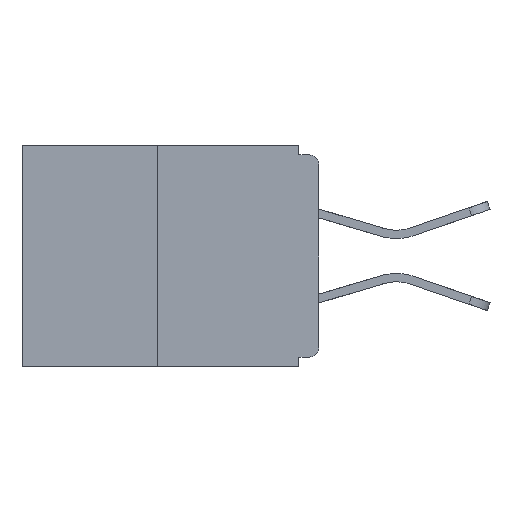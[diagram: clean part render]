
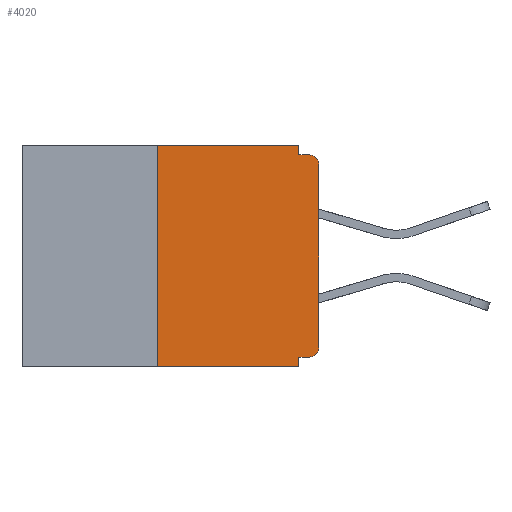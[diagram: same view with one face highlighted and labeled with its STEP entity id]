
A CAD part, left-side view. The second image highlights one B-rep face of the part: STEP entity #4020.
In plain terms, the highlighted planar face has unit normal (-1, 0, 0).
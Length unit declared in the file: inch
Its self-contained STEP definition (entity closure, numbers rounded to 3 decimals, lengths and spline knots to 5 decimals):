
#29 = VERTEX_POINT ( 'NONE', #1509 ) ;
#226 = DIRECTION ( 'NONE',  ( -1., 0., 0. ) ) ;
#231 = CARTESIAN_POINT ( 'NONE',  ( 0., 0.46, -0.343 ) ) ;
#475 = ORIENTED_EDGE ( 'NONE', *, *, #24253, .T. ) ;
#1274 = CARTESIAN_POINT ( 'NONE',  ( 0., 0., -0.015 ) ) ;
#1509 = CARTESIAN_POINT ( 'NONE',  ( 0., 0.015, -0.328 ) ) ;
#2218 = EDGE_CURVE ( 'NONE', #24492, #15950, #18961, .T. ) ;
#2872 = ORIENTED_EDGE ( 'NONE', *, *, #11935, .F. ) ;
#3116 = CARTESIAN_POINT ( 'NONE',  ( 0., 0.25, 0. ) ) ;
#3188 = CARTESIAN_POINT ( 'NONE',  ( 0., 0.25, 0. ) ) ;
#3460 = CARTESIAN_POINT ( 'NONE',  ( 0., 0.46, 0. ) ) ;
#3694 = DIRECTION ( 'NONE',  ( 0., 0., -1. ) ) ;
#4020 = ADVANCED_FACE ( 'NONE', ( #11728 ), #17610, .F. ) ;
#4146 = ORIENTED_EDGE ( 'NONE', *, *, #2218, .T. ) ;
#4351 = LINE ( 'NONE', #231, #6164 ) ;
#4354 = VERTEX_POINT ( 'NONE', #24860 ) ;
#5093 = CARTESIAN_POINT ( 'NONE',  ( 0., 0., -0.03 ) ) ;
#5268 = VECTOR ( 'NONE', #15161, 39.37008 ) ;
#5299 = LINE ( 'NONE', #11426, #5268 ) ;
#6164 = VECTOR ( 'NONE', #14494, 39.37008 ) ;
#6224 = CARTESIAN_POINT ( 'NONE',  ( 0., 0.25, -0.343 ) ) ;
#6852 = CARTESIAN_POINT ( 'NONE',  ( 0., 0., -0.328 ) ) ;
#7406 = LINE ( 'NONE', #1274, #23758 ) ;
#8199 = AXIS2_PLACEMENT_3D ( 'NONE', #9554, #17710, #3694 ) ;
#9290 = EDGE_CURVE ( 'NONE', #18717, #4354, #5299, .T. ) ;
#9554 = CARTESIAN_POINT ( 'NONE',  ( 0., 0.015, -0.313 ) ) ;
#9602 = VECTOR ( 'NONE', #14919, 39.37008 ) ;
#9695 = VERTEX_POINT ( 'NONE', #20982 ) ;
#9740 = DIRECTION ( 'NONE',  ( 0., 0., -1. ) ) ;
#9750 = CARTESIAN_POINT ( 'NONE',  ( 0., 0.031, 0. ) ) ;
#10863 = AXIS2_PLACEMENT_3D ( 'NONE', #3460, #19730, #9740 ) ;
#11277 = VERTEX_POINT ( 'NONE', #6224 ) ;
#11426 = CARTESIAN_POINT ( 'NONE',  ( 0., 0.031, 0. ) ) ;
#11728 = FACE_OUTER_BOUND ( 'NONE', #16400, .T. ) ;
#11935 = EDGE_CURVE ( 'NONE', #14613, #18717, #23924, .T. ) ;
#12484 = EDGE_CURVE ( 'NONE', #4354, #17338, #7406, .T. ) ;
#12827 = DIRECTION ( 'NONE',  ( 0., 0., 1. ) ) ;
#13901 = ORIENTED_EDGE ( 'NONE', *, *, #18565, .F. ) ;
#14037 = ORIENTED_EDGE ( 'NONE', *, *, #12484, .F. ) ;
#14494 = DIRECTION ( 'NONE',  ( 0., -1., 0. ) ) ;
#14555 = ORIENTED_EDGE ( 'NONE', *, *, #15553, .F. ) ;
#14613 = VERTEX_POINT ( 'NONE', #3188 ) ;
#14919 = DIRECTION ( 'NONE',  ( 0., 0., -1. ) ) ;
#15161 = DIRECTION ( 'NONE',  ( 0., 0., -1. ) ) ;
#15461 = CARTESIAN_POINT ( 'NONE',  ( 0., 0.031, -0.343 ) ) ;
#15553 = EDGE_CURVE ( 'NONE', #11277, #14613, #25410, .T. ) ;
#15651 = CARTESIAN_POINT ( 'NONE',  ( 0., 0.46, 0. ) ) ;
#15950 = VERTEX_POINT ( 'NONE', #5093 ) ;
#16400 = EDGE_LOOP ( 'NONE', ( #2872, #14555, #21274, #20410, #13901, #475, #4146, #19149, #14037, #20657 ) ) ;
#17338 = VERTEX_POINT ( 'NONE', #25361 ) ;
#17610 = PLANE ( 'NONE',  #10863 ) ;
#17710 = DIRECTION ( 'NONE',  ( -1., 0., 0. ) ) ;
#17884 = VECTOR ( 'NONE', #12827, 39.37008 ) ;
#17980 = EDGE_CURVE ( 'NONE', #11277, #20290, #4351, .T. ) ;
#18565 = EDGE_CURVE ( 'NONE', #29, #9695, #22722, .T. ) ;
#18610 = CARTESIAN_POINT ( 'NONE',  ( 0., 0.015, -0.03 ) ) ;
#18703 = DIRECTION ( 'NONE',  ( 0., 1., 0. ) ) ;
#18717 = VERTEX_POINT ( 'NONE', #9750 ) ;
#18866 = DIRECTION ( 'NONE',  ( 0., 0., -1. ) ) ;
#18961 = LINE ( 'NONE', #21228, #17884 ) ;
#19019 = EDGE_CURVE ( 'NONE', #9695, #20290, #23191, .T. ) ;
#19149 = ORIENTED_EDGE ( 'NONE', *, *, #21050, .T. ) ;
#19257 = DIRECTION ( 'NONE',  ( 0., 0., 1. ) ) ;
#19492 = DIRECTION ( 'NONE',  ( 0., -1., 0. ) ) ;
#19730 = DIRECTION ( 'NONE',  ( 1., 0., 0. ) ) ;
#20290 = VERTEX_POINT ( 'NONE', #23106 ) ;
#20410 = ORIENTED_EDGE ( 'NONE', *, *, #19019, .F. ) ;
#20657 = ORIENTED_EDGE ( 'NONE', *, *, #9290, .F. ) ;
#20959 = VECTOR ( 'NONE', #19492, 39.37008 ) ;
#20982 = CARTESIAN_POINT ( 'NONE',  ( 0., 0.031, -0.328 ) ) ;
#21050 = EDGE_CURVE ( 'NONE', #15950, #17338, #21751, .T. ) ;
#21228 = CARTESIAN_POINT ( 'NONE',  ( 0., 0., 0. ) ) ;
#21274 = ORIENTED_EDGE ( 'NONE', *, *, #17980, .T. ) ;
#21751 = CIRCLE ( 'NONE', #25164, 0.015 ) ;
#22661 = VECTOR ( 'NONE', #19257, 39.37008 ) ;
#22722 = LINE ( 'NONE', #6852, #24917 ) ;
#23106 = CARTESIAN_POINT ( 'NONE',  ( 0., 0.031, -0.343 ) ) ;
#23191 = LINE ( 'NONE', #15461, #9602 ) ;
#23389 = CARTESIAN_POINT ( 'NONE',  ( 0., 0., -0.313 ) ) ;
#23758 = VECTOR ( 'NONE', #23817, 39.37008 ) ;
#23817 = DIRECTION ( 'NONE',  ( 0., -1., 0. ) ) ;
#23924 = LINE ( 'NONE', #15651, #20959 ) ;
#24253 = EDGE_CURVE ( 'NONE', #29, #24492, #25680, .T. ) ;
#24492 = VERTEX_POINT ( 'NONE', #23389 ) ;
#24860 = CARTESIAN_POINT ( 'NONE',  ( 0., 0.031, -0.015 ) ) ;
#24917 = VECTOR ( 'NONE', #18703, 39.37008 ) ;
#25164 = AXIS2_PLACEMENT_3D ( 'NONE', #18610, #226, #18866 ) ;
#25361 = CARTESIAN_POINT ( 'NONE',  ( 0., 0.015, -0.015 ) ) ;
#25410 = LINE ( 'NONE', #3116, #22661 ) ;
#25680 = CIRCLE ( 'NONE', #8199, 0.015 ) ;
